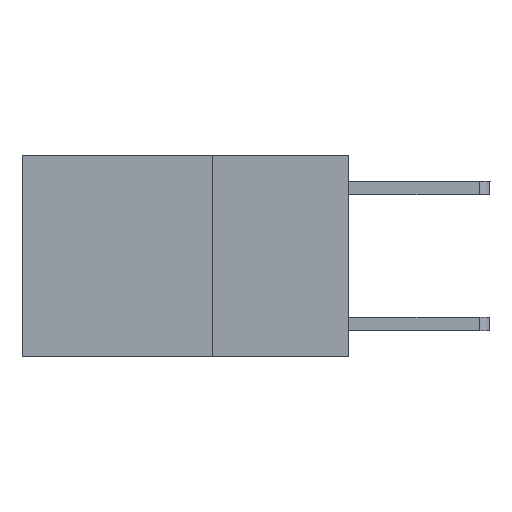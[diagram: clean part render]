
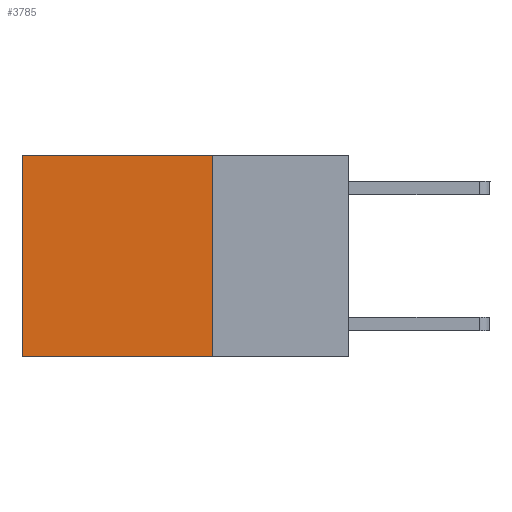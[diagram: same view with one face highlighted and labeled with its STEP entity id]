
A CAD part, left-side view. The second image highlights one B-rep face of the part: STEP entity #3785.
In plain terms, the highlighted planar face has unit normal (-1, 0, 0).
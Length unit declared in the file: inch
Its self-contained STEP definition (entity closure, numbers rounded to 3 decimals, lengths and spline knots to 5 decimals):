
#454 = ORIENTED_EDGE ( 'NONE', *, *, #1588, .T. ) ;
#905 = VERTEX_POINT ( 'NONE', #5659 ) ;
#1094 = DIRECTION ( 'NONE',  ( 0., 1., 0. ) ) ;
#1160 = VERTEX_POINT ( 'NONE', #8154 ) ;
#1576 = DIRECTION ( 'NONE',  ( 0., 0., -1. ) ) ;
#1588 = EDGE_CURVE ( 'NONE', #7576, #2886, #4574, .T. ) ;
#1711 = EDGE_CURVE ( 'NONE', #2886, #905, #3667, .T. ) ;
#2302 = LINE ( 'NONE', #7511, #7586 ) ;
#2369 = ORIENTED_EDGE ( 'NONE', *, *, #7499, .F. ) ;
#2846 = ORIENTED_EDGE ( 'NONE', *, *, #8499, .F. ) ;
#2886 = VERTEX_POINT ( 'NONE', #8781 ) ;
#3079 = EDGE_LOOP ( 'NONE', ( #8440, #2846, #2369, #454 ) ) ;
#3386 = DIRECTION ( 'NONE',  ( 0., 0., -1. ) ) ;
#3601 = VECTOR ( 'NONE', #3386, 39.37008 ) ;
#3667 = LINE ( 'NONE', #5638, #3601 ) ;
#3785 = ADVANCED_FACE ( 'NONE', ( #6947 ), #6244, .F. ) ;
#3970 = CARTESIAN_POINT ( 'NONE',  ( 0.2625, 0.25, 0. ) ) ;
#4574 = LINE ( 'NONE', #3970, #4790 ) ;
#4790 = VECTOR ( 'NONE', #1094, 39.37008 ) ;
#5638 = CARTESIAN_POINT ( 'NONE',  ( 0.2625, 0.6, 0. ) ) ;
#5659 = CARTESIAN_POINT ( 'NONE',  ( 0.2625, 0.6, -0.37 ) ) ;
#5738 = CARTESIAN_POINT ( 'NONE',  ( 0.2625, 0.25, 0. ) ) ;
#6041 = DIRECTION ( 'NONE',  ( 0., 0., -1. ) ) ;
#6244 = PLANE ( 'NONE',  #7250 ) ;
#6313 = DIRECTION ( 'NONE',  ( 1., 0., 0. ) ) ;
#6947 = FACE_OUTER_BOUND ( 'NONE', #3079, .T. ) ;
#6991 = CARTESIAN_POINT ( 'NONE',  ( 0.2625, 0.25, 0. ) ) ;
#7250 = AXIS2_PLACEMENT_3D ( 'NONE', #6991, #6313, #6041 ) ;
#7499 = EDGE_CURVE ( 'NONE', #7576, #1160, #9060, .T. ) ;
#7511 = CARTESIAN_POINT ( 'NONE',  ( 0.2625, 0.25, -0.37 ) ) ;
#7576 = VERTEX_POINT ( 'NONE', #8623 ) ;
#7586 = VECTOR ( 'NONE', #8264, 39.37008 ) ;
#8154 = CARTESIAN_POINT ( 'NONE',  ( 0.2625, 0.25, -0.37 ) ) ;
#8264 = DIRECTION ( 'NONE',  ( 0., 1., 0. ) ) ;
#8440 = ORIENTED_EDGE ( 'NONE', *, *, #1711, .T. ) ;
#8499 = EDGE_CURVE ( 'NONE', #1160, #905, #2302, .T. ) ;
#8623 = CARTESIAN_POINT ( 'NONE',  ( 0.2625, 0.25, 0. ) ) ;
#8781 = CARTESIAN_POINT ( 'NONE',  ( 0.2625, 0.6, 0. ) ) ;
#8880 = VECTOR ( 'NONE', #1576, 39.37008 ) ;
#9060 = LINE ( 'NONE', #5738, #8880 ) ;
